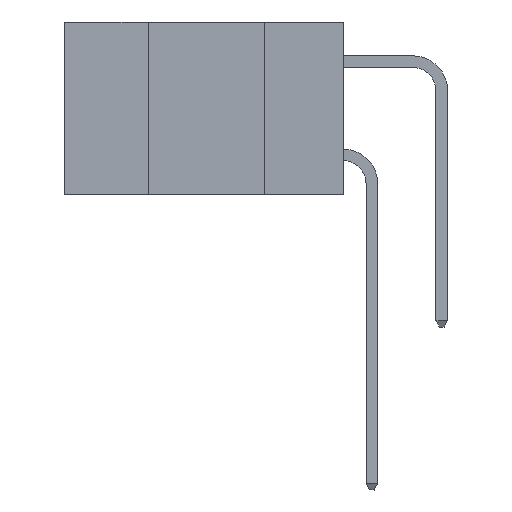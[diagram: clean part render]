
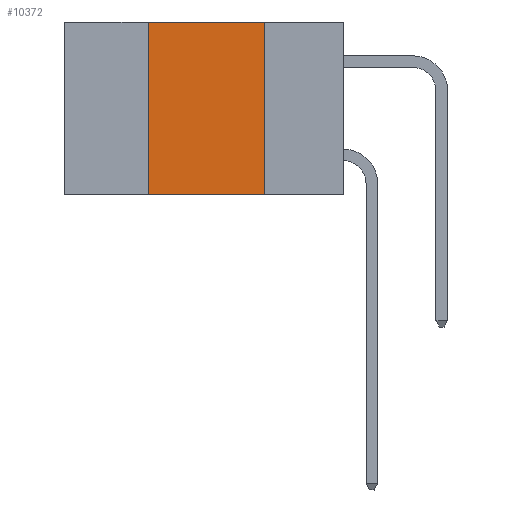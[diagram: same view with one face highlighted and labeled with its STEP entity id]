
A CAD part, left-side view. The second image highlights one B-rep face of the part: STEP entity #10372.
In plain terms, the highlighted planar face has unit normal (-1, 0, 0).
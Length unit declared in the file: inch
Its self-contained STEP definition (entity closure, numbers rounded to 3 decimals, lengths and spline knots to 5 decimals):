
#846 = VERTEX_POINT ( 'NONE', #2463 ) ;
#1235 = DIRECTION ( 'NONE',  ( 0., -1., 0. ) ) ;
#2174 = LINE ( 'NONE', #17057, #10709 ) ;
#2463 = CARTESIAN_POINT ( 'NONE',  ( 0., 0.42, -0.37 ) ) ;
#2682 = VECTOR ( 'NONE', #11498, 39.37008 ) ;
#2898 = CARTESIAN_POINT ( 'NONE',  ( 0., 0.42, 0. ) ) ;
#3211 = CARTESIAN_POINT ( 'NONE',  ( 0., 0.42, -0.37 ) ) ;
#3219 = PLANE ( 'NONE',  #4342 ) ;
#3931 = ORIENTED_EDGE ( 'NONE', *, *, #5095, .F. ) ;
#4056 = VERTEX_POINT ( 'NONE', #2898 ) ;
#4091 = CARTESIAN_POINT ( 'NONE',  ( 0., 0.6, -0.37 ) ) ;
#4250 = EDGE_CURVE ( 'NONE', #11950, #12032, #2174, .T. ) ;
#4342 = AXIS2_PLACEMENT_3D ( 'NONE', #17023, #14208, #4644 ) ;
#4599 = VECTOR ( 'NONE', #5775, 39.37008 ) ;
#4644 = DIRECTION ( 'NONE',  ( 0., 0., -1. ) ) ;
#5095 = EDGE_CURVE ( 'NONE', #846, #4056, #13128, .T. ) ;
#5428 = EDGE_LOOP ( 'NONE', ( #7659, #17621, #3931, #11261 ) ) ;
#5775 = DIRECTION ( 'NONE',  ( 0., -1., 0. ) ) ;
#6607 = EDGE_CURVE ( 'NONE', #4056, #11950, #9933, .T. ) ;
#7659 = ORIENTED_EDGE ( 'NONE', *, *, #4250, .F. ) ;
#8239 = CARTESIAN_POINT ( 'NONE',  ( 0., 0.17, -0.37 ) ) ;
#9106 = DIRECTION ( 'NONE',  ( 0., 0., -1. ) ) ;
#9933 = LINE ( 'NONE', #13890, #4599 ) ;
#10372 = ADVANCED_FACE ( 'NONE', ( #11506 ), #3219, .F. ) ;
#10456 = VECTOR ( 'NONE', #1235, 39.37008 ) ;
#10709 = VECTOR ( 'NONE', #9106, 39.37008 ) ;
#11261 = ORIENTED_EDGE ( 'NONE', *, *, #12106, .T. ) ;
#11498 = DIRECTION ( 'NONE',  ( 0., 0., 1. ) ) ;
#11506 = FACE_OUTER_BOUND ( 'NONE', #5428, .T. ) ;
#11950 = VERTEX_POINT ( 'NONE', #15940 ) ;
#12032 = VERTEX_POINT ( 'NONE', #8239 ) ;
#12106 = EDGE_CURVE ( 'NONE', #846, #12032, #13561, .T. ) ;
#13128 = LINE ( 'NONE', #3211, #2682 ) ;
#13561 = LINE ( 'NONE', #4091, #10456 ) ;
#13890 = CARTESIAN_POINT ( 'NONE',  ( 0., 0.6, 0. ) ) ;
#14208 = DIRECTION ( 'NONE',  ( 1., 0., 0. ) ) ;
#15940 = CARTESIAN_POINT ( 'NONE',  ( 0., 0.17, 0. ) ) ;
#17023 = CARTESIAN_POINT ( 'NONE',  ( 0., 0.6, 0. ) ) ;
#17057 = CARTESIAN_POINT ( 'NONE',  ( 0., 0.17, -0.37 ) ) ;
#17621 = ORIENTED_EDGE ( 'NONE', *, *, #6607, .F. ) ;
